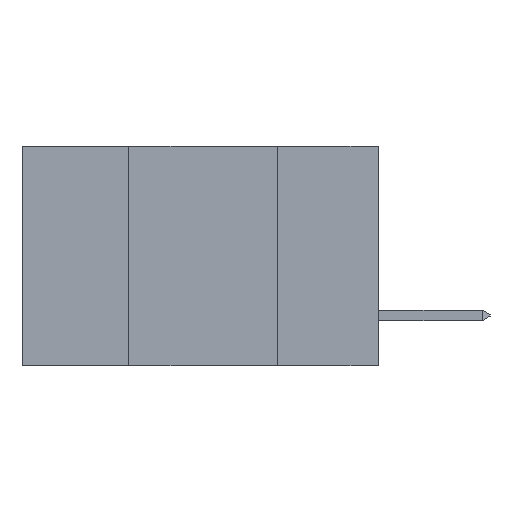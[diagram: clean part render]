
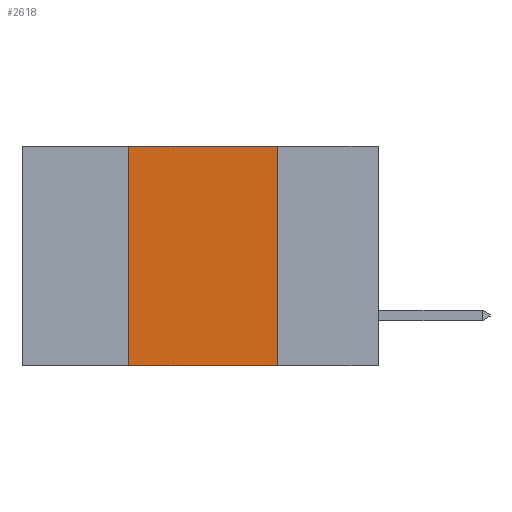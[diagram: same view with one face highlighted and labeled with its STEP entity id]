
A CAD part, left-side view. The second image highlights one B-rep face of the part: STEP entity #2618.
In plain terms, the highlighted planar face has unit normal (-1, 0, 0).
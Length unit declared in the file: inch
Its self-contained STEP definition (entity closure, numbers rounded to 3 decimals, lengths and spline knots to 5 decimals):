
#389 = LINE ( 'NONE', #11892, #8410 ) ;
#627 = VERTEX_POINT ( 'NONE', #18226 ) ;
#696 = CARTESIAN_POINT ( 'NONE',  ( 0., 0.17, 0. ) ) ;
#1779 = EDGE_CURVE ( 'NONE', #18320, #14654, #4522, .T. ) ;
#2311 = DIRECTION ( 'NONE',  ( 0., 0., -1. ) ) ;
#2618 = ADVANCED_FACE ( 'NONE', ( #14243 ), #11096, .F. ) ;
#3282 = LINE ( 'NONE', #12894, #15540 ) ;
#3712 = CARTESIAN_POINT ( 'NONE',  ( 0., 0.42, 0. ) ) ;
#4328 = EDGE_LOOP ( 'NONE', ( #19454, #13957, #9690, #6218 ) ) ;
#4522 = LINE ( 'NONE', #17796, #20243 ) ;
#4856 = DIRECTION ( 'NONE',  ( 0., -1., 0. ) ) ;
#5648 = CARTESIAN_POINT ( 'NONE',  ( 0., 0.6, 0. ) ) ;
#5706 = EDGE_CURVE ( 'NONE', #10329, #627, #3282, .T. ) ;
#6218 = ORIENTED_EDGE ( 'NONE', *, *, #1779, .T. ) ;
#8410 = VECTOR ( 'NONE', #13505, 39.37008 ) ;
#8813 = DIRECTION ( 'NONE',  ( 1., 0., 0. ) ) ;
#8950 = LINE ( 'NONE', #696, #13696 ) ;
#9690 = ORIENTED_EDGE ( 'NONE', *, *, #20135, .F. ) ;
#10329 = VERTEX_POINT ( 'NONE', #3712 ) ;
#11051 = DIRECTION ( 'NONE',  ( 0., -1., 0. ) ) ;
#11096 = PLANE ( 'NONE',  #15091 ) ;
#11570 = CARTESIAN_POINT ( 'NONE',  ( 0., 0.42, -0.37 ) ) ;
#11776 = CARTESIAN_POINT ( 'NONE',  ( 0., 0.17, -0.37 ) ) ;
#11892 = CARTESIAN_POINT ( 'NONE',  ( 0., 0.42, 0. ) ) ;
#12894 = CARTESIAN_POINT ( 'NONE',  ( 0., 0.6, 0. ) ) ;
#13505 = DIRECTION ( 'NONE',  ( 0., 0., 1. ) ) ;
#13696 = VECTOR ( 'NONE', #2311, 39.37008 ) ;
#13957 = ORIENTED_EDGE ( 'NONE', *, *, #5706, .F. ) ;
#14243 = FACE_OUTER_BOUND ( 'NONE', #4328, .T. ) ;
#14629 = DIRECTION ( 'NONE',  ( 0., 0., -1. ) ) ;
#14654 = VERTEX_POINT ( 'NONE', #11776 ) ;
#15091 = AXIS2_PLACEMENT_3D ( 'NONE', #5648, #8813, #14629 ) ;
#15540 = VECTOR ( 'NONE', #4856, 39.37008 ) ;
#17136 = EDGE_CURVE ( 'NONE', #627, #14654, #8950, .T. ) ;
#17796 = CARTESIAN_POINT ( 'NONE',  ( 0., 0.6, -0.37 ) ) ;
#18226 = CARTESIAN_POINT ( 'NONE',  ( 0., 0.17, 0. ) ) ;
#18320 = VERTEX_POINT ( 'NONE', #11570 ) ;
#19454 = ORIENTED_EDGE ( 'NONE', *, *, #17136, .F. ) ;
#20135 = EDGE_CURVE ( 'NONE', #18320, #10329, #389, .T. ) ;
#20243 = VECTOR ( 'NONE', #11051, 39.37008 ) ;
